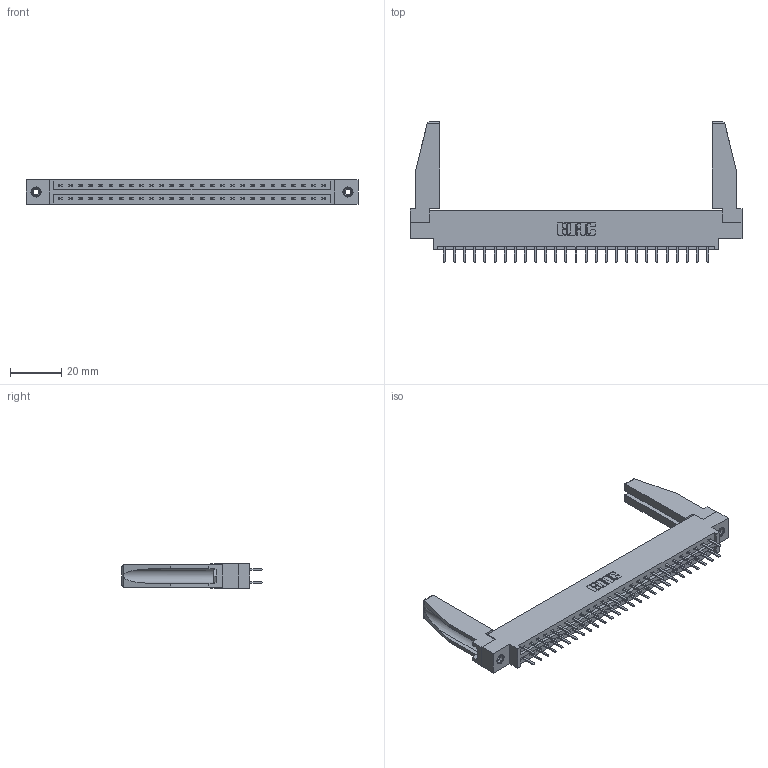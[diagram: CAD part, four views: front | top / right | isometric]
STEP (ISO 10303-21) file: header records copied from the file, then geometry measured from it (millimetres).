
FILE_DESCRIPTION (( 'STEP AP203' ), '1' );
FILE_NAME ('387-054-520-878.STEP', '2019-10-19T04:25:04', ( '' ), ( '' ), 'SwSTEP 2.0', 'SolidWorks 2016', '' );
FILE_SCHEMA (( 'CONFIG_CONTROL_DESIGN' ));
Length unit declared in the file: inch
Products named in the file (5): 345-292-001_345-293-120; 307-220-078; 337 Part_0.170 Offset - 0.156 Dia-TI; 345-250-001_345-250-001-102; 387-054-520-878
Assembly tree (59 placements, depth 2):
  387-054-520-878
    337 Part_0.170 Offset - 0.156 Dia-TI
    345-292-001_345-293-120  x54
    345-250-001_345-250-001-102  x2
    307-220-078  x2
Bounding box: 130 x 54.82 x 9.4 mm (x, y, z)
Volume: 17352.6 mm3; surface area: 18827.5 mm2
Topology: 59 solids, 59 shells, 3380 faces, 9779 edges, 6366 vertices
Faces by surface type: plane 2318, cylinder 1046, cone 12, torus 4
Entity records: 25560 total; most frequent: CARTESIAN_POINT 4332, ORIENTED_EDGE 4212, DIRECTION 3706, EDGE_CURVE 2106, VECTOR 1936, LINE 1936, VERTEX_POINT 1396, AXIS2_PLACEMENT_3D 885
